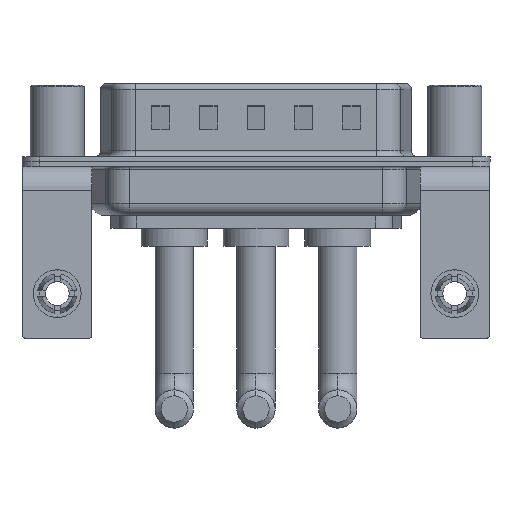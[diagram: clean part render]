
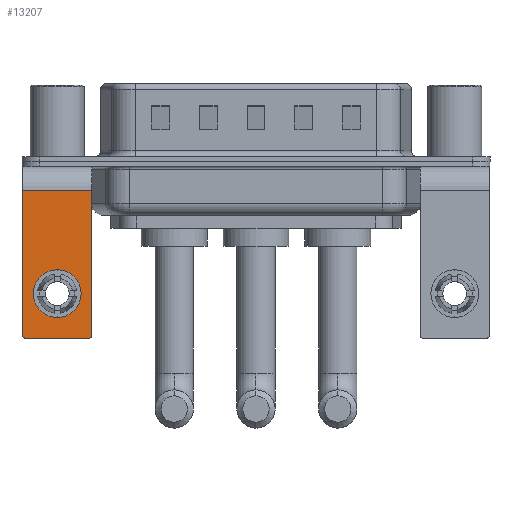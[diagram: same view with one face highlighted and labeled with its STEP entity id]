
A CAD part, front view. The second image highlights one B-rep face of the part: STEP entity #13207.
In plain terms, the highlighted planar face has unit normal (0, -1, 0).
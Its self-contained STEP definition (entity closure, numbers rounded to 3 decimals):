
#172 = VECTOR ( 'NONE', #11242, 1000. ) ;
#197 = EDGE_CURVE ( 'NONE', #19061, #16652, #14254, .T. ) ;
#487 = CARTESIAN_POINT ( 'NONE',  ( -2.65, -6.25, -14.8 ) ) ;
#759 = FACE_BOUND ( 'NONE', #9880, .T. ) ;
#860 = EDGE_CURVE ( 'NONE', #15158, #3205, #9995, .T. ) ;
#916 = DIRECTION ( 'NONE',  ( 0., 1., 0. ) ) ;
#1853 = DIRECTION ( 'NONE',  ( 0., 0., -1. ) ) ;
#2382 = ORIENTED_EDGE ( 'NONE', *, *, #12010, .T. ) ;
#2589 = VERTEX_POINT ( 'NONE', #487 ) ;
#2673 = DIRECTION ( 'NONE',  ( 0., 0., 1. ) ) ;
#2683 = VECTOR ( 'NONE', #1853, 1000. ) ;
#2861 = DIRECTION ( 'NONE',  ( 0., 1., 0. ) ) ;
#2950 = CARTESIAN_POINT ( 'NONE',  ( 2.9, -6.25, -2.4 ) ) ;
#3205 = VERTEX_POINT ( 'NONE', #5691 ) ;
#3747 = LINE ( 'NONE', #15608, #172 ) ;
#3842 = DIRECTION ( 'NONE',  ( 0., 0., 1. ) ) ;
#3867 = ORIENTED_EDGE ( 'NONE', *, *, #860, .T. ) ;
#3915 = CARTESIAN_POINT ( 'NONE',  ( 0., -6.25, -11.07 ) ) ;
#4592 = DIRECTION ( 'NONE',  ( -1., 0., 0. ) ) ;
#5691 = CARTESIAN_POINT ( 'NONE',  ( 0., -6.25, -9.07 ) ) ;
#6048 = LINE ( 'NONE', #10354, #6131 ) ;
#6131 = VECTOR ( 'NONE', #4592, 1000. ) ;
#6520 = CARTESIAN_POINT ( 'NONE',  ( -2.9, -6.25, -2.4 ) ) ;
#7260 = VERTEX_POINT ( 'NONE', #13150 ) ;
#7322 = CARTESIAN_POINT ( 'NONE',  ( 0., -6.25, -11.07 ) ) ;
#7384 = CARTESIAN_POINT ( 'NONE',  ( -2.9, -6.25, -2.4 ) ) ;
#7560 = DIRECTION ( 'NONE',  ( 0., 0., 1. ) ) ;
#8105 = CARTESIAN_POINT ( 'NONE',  ( -2.9, -6.25, -14.55 ) ) ;
#8727 = EDGE_CURVE ( 'NONE', #12927, #17301, #15167, .T. ) ;
#8890 = DIRECTION ( 'NONE',  ( 0., 0., 1. ) ) ;
#9035 = CARTESIAN_POINT ( 'NONE',  ( 2.9, -6.25, -14.55 ) ) ;
#9880 = EDGE_LOOP ( 'NONE', ( #3867, #11462 ) ) ;
#9928 = AXIS2_PLACEMENT_3D ( 'NONE', #2950, #2861, #2673 ) ;
#9995 = CIRCLE ( 'NONE', #14342, 2. ) ;
#10176 = CIRCLE ( 'NONE', #17310, 0.25 ) ;
#10203 = DIRECTION ( 'NONE',  ( 0., -1., 0. ) ) ;
#10354 = CARTESIAN_POINT ( 'NONE',  ( 2.9, -6.25, -2.4 ) ) ;
#10455 = AXIS2_PLACEMENT_3D ( 'NONE', #7322, #13258, #8890 ) ;
#10458 = EDGE_CURVE ( 'NONE', #7260, #16652, #3747, .T. ) ;
#10469 = ORIENTED_EDGE ( 'NONE', *, *, #18799, .F. ) ;
#10805 = AXIS2_PLACEMENT_3D ( 'NONE', #11538, #17355, #3842 ) ;
#11242 = DIRECTION ( 'NONE',  ( 0., 0., -1. ) ) ;
#11307 = DIRECTION ( 'NONE',  ( -1., 0., 0. ) ) ;
#11462 = ORIENTED_EDGE ( 'NONE', *, *, #15854, .T. ) ;
#11538 = CARTESIAN_POINT ( 'NONE',  ( 2.65, -6.25, -14.55 ) ) ;
#11555 = ORIENTED_EDGE ( 'NONE', *, *, #16755, .T. ) ;
#12010 = EDGE_CURVE ( 'NONE', #7260, #12927, #6048, .T. ) ;
#12696 = DIRECTION ( 'NONE',  ( 0., 0., 1. ) ) ;
#12728 = CARTESIAN_POINT ( 'NONE',  ( 0., -6.25, -13.07 ) ) ;
#12772 = CARTESIAN_POINT ( 'NONE',  ( 2.9, -6.25, -14.8 ) ) ;
#12927 = VERTEX_POINT ( 'NONE', #7384 ) ;
#13150 = CARTESIAN_POINT ( 'NONE',  ( 2.9, -6.25, -2.4 ) ) ;
#13207 = ADVANCED_FACE ( 'NONE', ( #759, #18541 ), #15989, .F. ) ;
#13258 = DIRECTION ( 'NONE',  ( 0., 1., 0. ) ) ;
#13347 = ORIENTED_EDGE ( 'NONE', *, *, #10458, .F. ) ;
#14254 = CIRCLE ( 'NONE', #10805, 0.25 ) ;
#14342 = AXIS2_PLACEMENT_3D ( 'NONE', #3915, #916, #12696 ) ;
#14660 = CARTESIAN_POINT ( 'NONE',  ( -2.65, -6.25, -14.55 ) ) ;
#15158 = VERTEX_POINT ( 'NONE', #12728 ) ;
#15167 = LINE ( 'NONE', #6520, #2683 ) ;
#15469 = VECTOR ( 'NONE', #11307, 1000. ) ;
#15608 = CARTESIAN_POINT ( 'NONE',  ( 2.9, -6.25, -2.4 ) ) ;
#15854 = EDGE_CURVE ( 'NONE', #3205, #15158, #18840, .T. ) ;
#15989 = PLANE ( 'NONE',  #9928 ) ;
#16652 = VERTEX_POINT ( 'NONE', #9035 ) ;
#16755 = EDGE_CURVE ( 'NONE', #17301, #2589, #10176, .T. ) ;
#17043 = ORIENTED_EDGE ( 'NONE', *, *, #197, .T. ) ;
#17301 = VERTEX_POINT ( 'NONE', #8105 ) ;
#17310 = AXIS2_PLACEMENT_3D ( 'NONE', #14660, #10203, #7560 ) ;
#17355 = DIRECTION ( 'NONE',  ( 0., -1., 0. ) ) ;
#17751 = LINE ( 'NONE', #12772, #15469 ) ;
#17907 = EDGE_LOOP ( 'NONE', ( #18791, #11555, #10469, #17043, #13347, #2382 ) ) ;
#18033 = CARTESIAN_POINT ( 'NONE',  ( 2.65, -6.25, -14.8 ) ) ;
#18541 = FACE_OUTER_BOUND ( 'NONE', #17907, .T. ) ;
#18791 = ORIENTED_EDGE ( 'NONE', *, *, #8727, .T. ) ;
#18799 = EDGE_CURVE ( 'NONE', #19061, #2589, #17751, .T. ) ;
#18840 = CIRCLE ( 'NONE', #10455, 2. ) ;
#19061 = VERTEX_POINT ( 'NONE', #18033 ) ;
